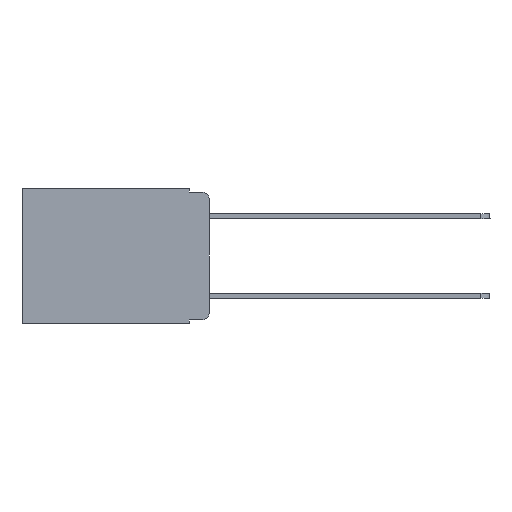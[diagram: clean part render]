
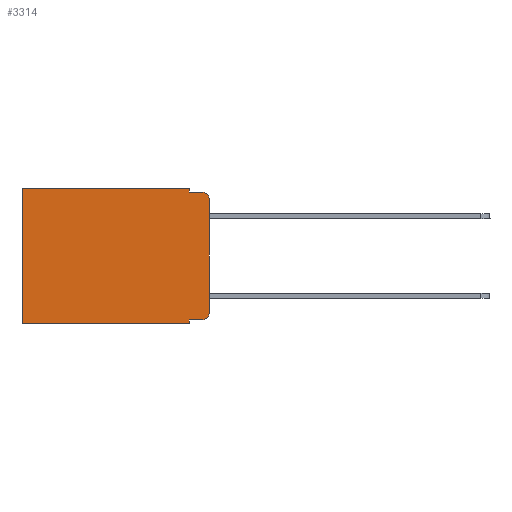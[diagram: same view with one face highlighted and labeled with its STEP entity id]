
A CAD part, left-side view. The second image highlights one B-rep face of the part: STEP entity #3314.
In plain terms, the highlighted planar face has unit normal (-1, 0, 0).
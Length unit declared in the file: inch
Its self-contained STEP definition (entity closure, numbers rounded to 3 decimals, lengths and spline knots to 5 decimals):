
#449 = DIRECTION ( 'NONE',  ( 0., 0., -1. ) ) ;
#455 = CARTESIAN_POINT ( 'NONE',  ( 0.298, 0.02, -0.313 ) ) ;
#523 = VECTOR ( 'NONE', #19003, 39.37008 ) ;
#1298 = LINE ( 'NONE', #8416, #14174 ) ;
#1548 = EDGE_CURVE ( 'NONE', #20308, #2487, #2970, .T. ) ;
#1830 = CARTESIAN_POINT ( 'NONE',  ( 0.298, 0.02, -0.01 ) ) ;
#1875 = EDGE_CURVE ( 'NONE', #3315, #5280, #21028, .T. ) ;
#2004 = ORIENTED_EDGE ( 'NONE', *, *, #7321, .T. ) ;
#2165 = VECTOR ( 'NONE', #10083, 39.37008 ) ;
#2267 = DIRECTION ( 'NONE',  ( 0., 0., -1. ) ) ;
#2286 = CIRCLE ( 'NONE', #20833, 0.02 ) ;
#2487 = VERTEX_POINT ( 'NONE', #9917 ) ;
#2970 = LINE ( 'NONE', #9010, #20268 ) ;
#3314 = ADVANCED_FACE ( 'NONE', ( #10919 ), #5424, .F. ) ;
#3315 = VERTEX_POINT ( 'NONE', #13889 ) ;
#3520 = DIRECTION ( 'NONE',  ( 1., 0., 0. ) ) ;
#3949 = EDGE_CURVE ( 'NONE', #7901, #9559, #6937, .T. ) ;
#4840 = EDGE_CURVE ( 'NONE', #9605, #8034, #21581, .T. ) ;
#4877 = DIRECTION ( 'NONE',  ( 0., 0., -1. ) ) ;
#5280 = VERTEX_POINT ( 'NONE', #20671 ) ;
#5424 = PLANE ( 'NONE',  #17687 ) ;
#5617 = ORIENTED_EDGE ( 'NONE', *, *, #6763, .F. ) ;
#6763 = EDGE_CURVE ( 'NONE', #9559, #8636, #11055, .T. ) ;
#6937 = LINE ( 'NONE', #9263, #13229 ) ;
#7260 = CARTESIAN_POINT ( 'NONE',  ( 0.298, 0., 0. ) ) ;
#7321 = EDGE_CURVE ( 'NONE', #19052, #5280, #1298, .T. ) ;
#7778 = CARTESIAN_POINT ( 'NONE',  ( 0.298, 0.473, 0. ) ) ;
#7901 = VERTEX_POINT ( 'NONE', #19853 ) ;
#8034 = VERTEX_POINT ( 'NONE', #8632 ) ;
#8097 = EDGE_CURVE ( 'NONE', #9605, #8636, #2286, .T. ) ;
#8416 = CARTESIAN_POINT ( 'NONE',  ( 0.298, 0.473, 0. ) ) ;
#8522 = VECTOR ( 'NONE', #2267, 39.37008 ) ;
#8632 = CARTESIAN_POINT ( 'NONE',  ( 0.298, 0., -0.313 ) ) ;
#8636 = VERTEX_POINT ( 'NONE', #1830 ) ;
#9010 = CARTESIAN_POINT ( 'NONE',  ( 0.298, 0.051, -0.333 ) ) ;
#9169 = DIRECTION ( 'NONE',  ( 0., 0., -1. ) ) ;
#9263 = CARTESIAN_POINT ( 'NONE',  ( 0.298, 0.051, 0. ) ) ;
#9559 = VERTEX_POINT ( 'NONE', #16794 ) ;
#9605 = VERTEX_POINT ( 'NONE', #10538 ) ;
#9917 = CARTESIAN_POINT ( 'NONE',  ( 0.298, 0.02, -0.333 ) ) ;
#10083 = DIRECTION ( 'NONE',  ( 0., 1., 0. ) ) ;
#10538 = CARTESIAN_POINT ( 'NONE',  ( 0.298, 0., -0.03 ) ) ;
#10593 = DIRECTION ( 'NONE',  ( -1., 0., 0. ) ) ;
#10689 = DIRECTION ( 'NONE',  ( 0., -1., 0. ) ) ;
#10714 = ORIENTED_EDGE ( 'NONE', *, *, #20335, .T. ) ;
#10871 = EDGE_LOOP ( 'NONE', ( #12411, #15613, #5617, #16326, #10714, #2004, #11885, #20827, #16841, #16050 ) ) ;
#10919 = FACE_OUTER_BOUND ( 'NONE', #10871, .T. ) ;
#11055 = LINE ( 'NONE', #13985, #523 ) ;
#11356 = CARTESIAN_POINT ( 'NONE',  ( 0.298, 0.051, -0.333 ) ) ;
#11505 = CARTESIAN_POINT ( 'NONE',  ( 0.298, 0., -0.343 ) ) ;
#11885 = ORIENTED_EDGE ( 'NONE', *, *, #1875, .F. ) ;
#12166 = DIRECTION ( 'NONE',  ( 0., 0., -1. ) ) ;
#12411 = ORIENTED_EDGE ( 'NONE', *, *, #4840, .F. ) ;
#13229 = VECTOR ( 'NONE', #19110, 39.37008 ) ;
#13815 = DIRECTION ( 'NONE',  ( 0., 0., -1. ) ) ;
#13889 = CARTESIAN_POINT ( 'NONE',  ( 0.298, 0.051, -0.343 ) ) ;
#13985 = CARTESIAN_POINT ( 'NONE',  ( 0.298, 0.051, -0.01 ) ) ;
#14174 = VECTOR ( 'NONE', #4877, 39.37008 ) ;
#14266 = AXIS2_PLACEMENT_3D ( 'NONE', #455, #18706, #12166 ) ;
#15613 = ORIENTED_EDGE ( 'NONE', *, *, #8097, .T. ) ;
#16050 = ORIENTED_EDGE ( 'NONE', *, *, #21478, .T. ) ;
#16326 = ORIENTED_EDGE ( 'NONE', *, *, #3949, .F. ) ;
#16421 = DIRECTION ( 'NONE',  ( 0., 1., 0. ) ) ;
#16794 = CARTESIAN_POINT ( 'NONE',  ( 0.298, 0.051, -0.01 ) ) ;
#16841 = ORIENTED_EDGE ( 'NONE', *, *, #1548, .T. ) ;
#17468 = CARTESIAN_POINT ( 'NONE',  ( 0.298, 0.051, 0. ) ) ;
#17663 = EDGE_CURVE ( 'NONE', #20308, #3315, #19121, .T. ) ;
#17687 = AXIS2_PLACEMENT_3D ( 'NONE', #18543, #3520, #13815 ) ;
#17810 = VECTOR ( 'NONE', #9169, 39.37008 ) ;
#18234 = VECTOR ( 'NONE', #16421, 39.37008 ) ;
#18543 = CARTESIAN_POINT ( 'NONE',  ( 0.298, 0., 0. ) ) ;
#18706 = DIRECTION ( 'NONE',  ( -1., 0., 0. ) ) ;
#18837 = CARTESIAN_POINT ( 'NONE',  ( 0.298, 0.02, -0.03 ) ) ;
#19003 = DIRECTION ( 'NONE',  ( 0., -1., 0. ) ) ;
#19052 = VERTEX_POINT ( 'NONE', #7778 ) ;
#19110 = DIRECTION ( 'NONE',  ( 0., 0., -1. ) ) ;
#19121 = LINE ( 'NONE', #17468, #17810 ) ;
#19853 = CARTESIAN_POINT ( 'NONE',  ( 0.298, 0.051, 0. ) ) ;
#20268 = VECTOR ( 'NONE', #10689, 39.37008 ) ;
#20308 = VERTEX_POINT ( 'NONE', #11356 ) ;
#20335 = EDGE_CURVE ( 'NONE', #7901, #19052, #21117, .T. ) ;
#20671 = CARTESIAN_POINT ( 'NONE',  ( 0.298, 0.473, -0.343 ) ) ;
#20827 = ORIENTED_EDGE ( 'NONE', *, *, #17663, .F. ) ;
#20833 = AXIS2_PLACEMENT_3D ( 'NONE', #18837, #10593, #449 ) ;
#21028 = LINE ( 'NONE', #11505, #2165 ) ;
#21117 = LINE ( 'NONE', #21195, #18234 ) ;
#21195 = CARTESIAN_POINT ( 'NONE',  ( 0.298, 0., 0. ) ) ;
#21478 = EDGE_CURVE ( 'NONE', #2487, #8034, #21606, .T. ) ;
#21581 = LINE ( 'NONE', #7260, #8522 ) ;
#21606 = CIRCLE ( 'NONE', #14266, 0.02 ) ;
